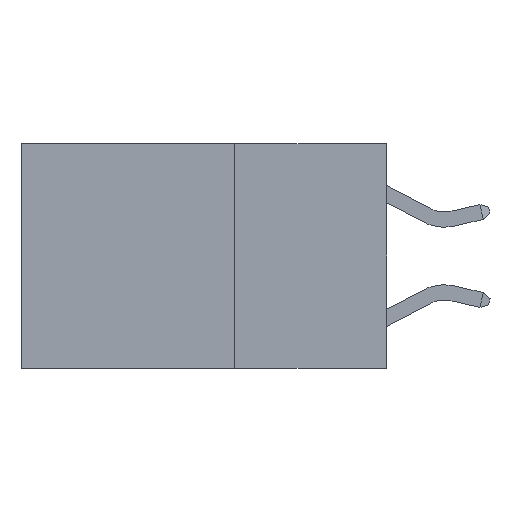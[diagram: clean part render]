
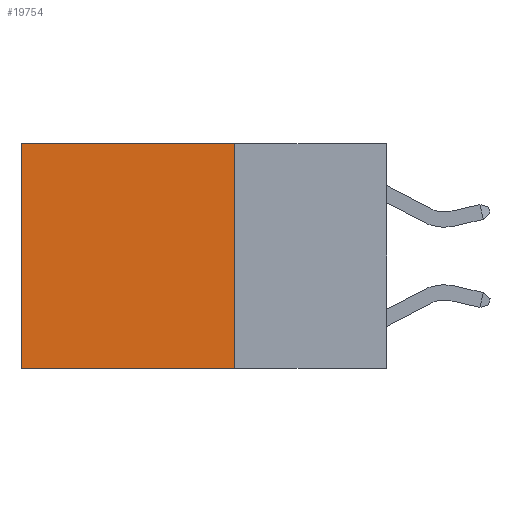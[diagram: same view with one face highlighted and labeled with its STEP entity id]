
A CAD part, left-side view. The second image highlights one B-rep face of the part: STEP entity #19754.
In plain terms, the highlighted planar face has unit normal (-1, 0, 0).
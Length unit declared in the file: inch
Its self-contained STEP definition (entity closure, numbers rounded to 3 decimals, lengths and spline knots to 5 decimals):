
#51 = CARTESIAN_POINT ( 'NONE',  ( 0.2625, 0.25, -0.37 ) ) ;
#123 = ORIENTED_EDGE ( 'NONE', *, *, #20092, .F. ) ;
#331 = CARTESIAN_POINT ( 'NONE',  ( 0.2625, 0.25, 0. ) ) ;
#3258 = VECTOR ( 'NONE', #3756, 39.37008 ) ;
#3261 = CARTESIAN_POINT ( 'NONE',  ( 0.2625, 0.6, 0. ) ) ;
#3756 = DIRECTION ( 'NONE',  ( 0., 0., -1. ) ) ;
#3954 = PLANE ( 'NONE',  #13605 ) ;
#4235 = VERTEX_POINT ( 'NONE', #11853 ) ;
#5427 = LINE ( 'NONE', #22322, #19197 ) ;
#6014 = ORIENTED_EDGE ( 'NONE', *, *, #10648, .T. ) ;
#6289 = EDGE_CURVE ( 'NONE', #7095, #4235, #7770, .T. ) ;
#6494 = VECTOR ( 'NONE', #10265, 39.37008 ) ;
#7095 = VERTEX_POINT ( 'NONE', #8657 ) ;
#7385 = DIRECTION ( 'NONE',  ( 1., 0., 0. ) ) ;
#7770 = LINE ( 'NONE', #331, #3258 ) ;
#8657 = CARTESIAN_POINT ( 'NONE',  ( 0.2625, 0.25, 0. ) ) ;
#9728 = ORIENTED_EDGE ( 'NONE', *, *, #6289, .F. ) ;
#10265 = DIRECTION ( 'NONE',  ( 0., 1., 0. ) ) ;
#10597 = DIRECTION ( 'NONE',  ( 0., 0., -1. ) ) ;
#10648 = EDGE_CURVE ( 'NONE', #15260, #21066, #12452, .T. ) ;
#10791 = ORIENTED_EDGE ( 'NONE', *, *, #18126, .T. ) ;
#11536 = LINE ( 'NONE', #51, #6494 ) ;
#11709 = DIRECTION ( 'NONE',  ( 0., 1., 0. ) ) ;
#11853 = CARTESIAN_POINT ( 'NONE',  ( 0.2625, 0.25, -0.37 ) ) ;
#12452 = LINE ( 'NONE', #17491, #17636 ) ;
#13605 = AXIS2_PLACEMENT_3D ( 'NONE', #17700, #7385, #19502 ) ;
#14300 = CARTESIAN_POINT ( 'NONE',  ( 0.2625, 0.6, -0.37 ) ) ;
#15260 = VERTEX_POINT ( 'NONE', #3261 ) ;
#17491 = CARTESIAN_POINT ( 'NONE',  ( 0.2625, 0.6, 0. ) ) ;
#17636 = VECTOR ( 'NONE', #10597, 39.37008 ) ;
#17700 = CARTESIAN_POINT ( 'NONE',  ( 0.2625, 0.25, 0. ) ) ;
#18126 = EDGE_CURVE ( 'NONE', #7095, #15260, #5427, .T. ) ;
#19197 = VECTOR ( 'NONE', #11709, 39.37008 ) ;
#19502 = DIRECTION ( 'NONE',  ( 0., 0., -1. ) ) ;
#19754 = ADVANCED_FACE ( 'NONE', ( #20223 ), #3954, .F. ) ;
#20092 = EDGE_CURVE ( 'NONE', #4235, #21066, #11536, .T. ) ;
#20223 = FACE_OUTER_BOUND ( 'NONE', #20809, .T. ) ;
#20809 = EDGE_LOOP ( 'NONE', ( #6014, #123, #9728, #10791 ) ) ;
#21066 = VERTEX_POINT ( 'NONE', #14300 ) ;
#22322 = CARTESIAN_POINT ( 'NONE',  ( 0.2625, 0.25, 0. ) ) ;
